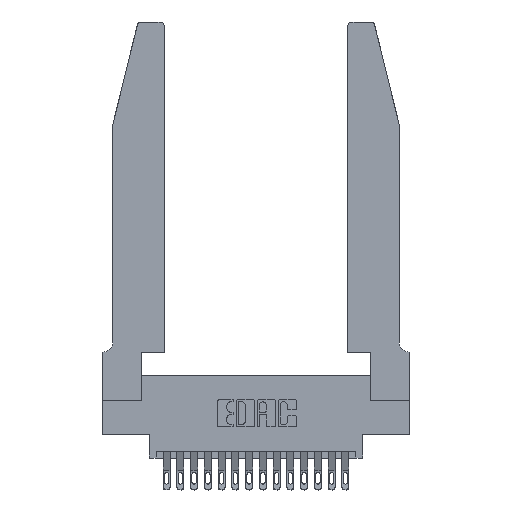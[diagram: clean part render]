
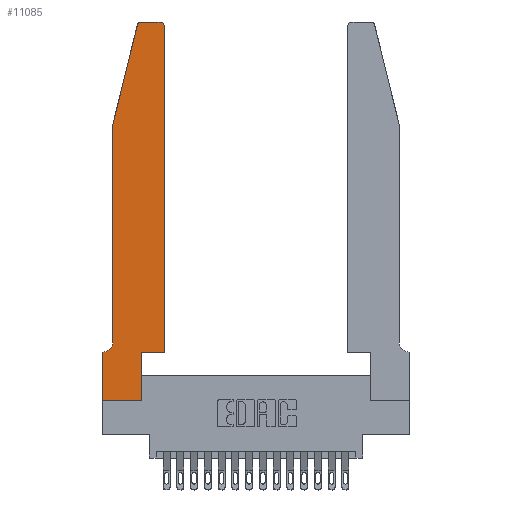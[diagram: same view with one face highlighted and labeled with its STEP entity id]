
A CAD part, top view. The second image highlights one B-rep face of the part: STEP entity #11085.
In plain terms, the highlighted planar face has unit normal (0, 0, 1).
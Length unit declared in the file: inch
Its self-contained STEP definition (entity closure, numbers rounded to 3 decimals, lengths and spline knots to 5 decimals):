
#4 = CARTESIAN_POINT ( 'NONE',  ( 0.4505, 2.72, 0.37 ) ) ;
#58 = CARTESIAN_POINT ( 'NONE',  ( 0.4505, 0.35, 0.37 ) ) ;
#345 = ORIENTED_EDGE ( 'NONE', *, *, #15492, .T. ) ;
#441 = DIRECTION ( 'NONE',  ( -1., 0., 0. ) ) ;
#541 = VERTEX_POINT ( 'NONE', #14167 ) ;
#592 = DIRECTION ( 'NONE',  ( 0., 1., 0. ) ) ;
#723 = CARTESIAN_POINT ( 'NONE',  ( 0.0055, 0.35, 0.37 ) ) ;
#910 = VERTEX_POINT ( 'NONE', #12138 ) ;
#1115 = AXIS2_PLACEMENT_3D ( 'NONE', #13196, #3932, #14712 ) ;
#1235 = DIRECTION ( 'NONE',  ( 1., 0., 0. ) ) ;
#1678 = CARTESIAN_POINT ( 'NONE',  ( 0., 0., 0.37 ) ) ;
#2380 = PLANE ( 'NONE',  #18724 ) ;
#2677 = LINE ( 'NONE', #18085, #17992 ) ;
#2682 = LINE ( 'NONE', #19079, #10477 ) ;
#2796 = EDGE_CURVE ( 'NONE', #14318, #12130, #13355, .T. ) ;
#2851 = DIRECTION ( 'NONE',  ( 0., 1., 0. ) ) ;
#2963 = EDGE_CURVE ( 'NONE', #10115, #4960, #7600, .T. ) ;
#3346 = DIRECTION ( 'NONE',  ( 1., 0., 0. ) ) ;
#3350 = EDGE_CURVE ( 'NONE', #5013, #13885, #16588, .T. ) ;
#3449 = CARTESIAN_POINT ( 'NONE',  ( 0.284, 2.75, 0.37 ) ) ;
#3913 = ORIENTED_EDGE ( 'NONE', *, *, #14777, .T. ) ;
#3932 = DIRECTION ( 'NONE',  ( 0., 0., -1. ) ) ;
#4013 = DIRECTION ( 'NONE',  ( 1., 0., 0. ) ) ;
#4354 = VECTOR ( 'NONE', #18451, 39.37008 ) ;
#4436 = VECTOR ( 'NONE', #9492, 39.37008 ) ;
#4551 = EDGE_CURVE ( 'NONE', #6329, #5013, #13321, .T. ) ;
#4612 = ORIENTED_EDGE ( 'NONE', *, *, #2963, .T. ) ;
#4767 = CARTESIAN_POINT ( 'NONE',  ( 0., 0.35, 0.37 ) ) ;
#4909 = ORIENTED_EDGE ( 'NONE', *, *, #10241, .T. ) ;
#4960 = VERTEX_POINT ( 'NONE', #723 ) ;
#5013 = VERTEX_POINT ( 'NONE', #8833 ) ;
#5078 = ORIENTED_EDGE ( 'NONE', *, *, #3350, .T. ) ;
#5857 = ORIENTED_EDGE ( 'NONE', *, *, #10189, .T. ) ;
#5964 = CARTESIAN_POINT ( 'NONE',  ( 0.284, 2.72, 0.37 ) ) ;
#6329 = VERTEX_POINT ( 'NONE', #3449 ) ;
#6366 = CARTESIAN_POINT ( 'NONE',  ( 0.0755, 0.35, 0.37 ) ) ;
#6390 = CARTESIAN_POINT ( 'NONE',  ( 0.4505, 0.35, 0.37 ) ) ;
#6743 = ORIENTED_EDGE ( 'NONE', *, *, #4551, .T. ) ;
#7114 = ORIENTED_EDGE ( 'NONE', *, *, #2796, .T. ) ;
#7282 = LINE ( 'NONE', #6390, #19296 ) ;
#7497 = DIRECTION ( 'NONE',  ( 1., 0., 0. ) ) ;
#7600 = CIRCLE ( 'NONE', #1115, 0.07 ) ;
#7942 = CARTESIAN_POINT ( 'NONE',  ( 0.0755, 2., 0.37 ) ) ;
#8217 = FACE_OUTER_BOUND ( 'NONE', #10931, .T. ) ;
#8408 = CARTESIAN_POINT ( 'NONE',  ( 0.0755, 2., 0.37 ) ) ;
#8461 = VERTEX_POINT ( 'NONE', #10868 ) ;
#8574 = VERTEX_POINT ( 'NONE', #58 ) ;
#8578 = CARTESIAN_POINT ( 'NONE',  ( 0.0755, 2., 0.37 ) ) ;
#8833 = CARTESIAN_POINT ( 'NONE',  ( 0.25487, 2.72718, 0.37 ) ) ;
#9206 = LINE ( 'NONE', #8578, #12765 ) ;
#9492 = DIRECTION ( 'NONE',  ( -0.239, -0.971, 0. ) ) ;
#9645 = VERTEX_POINT ( 'NONE', #4 ) ;
#9735 = VECTOR ( 'NONE', #15052, 39.37008 ) ;
#10003 = ORIENTED_EDGE ( 'NONE', *, *, #16224, .T. ) ;
#10101 = DIRECTION ( 'NONE',  ( 0., -1., 0. ) ) ;
#10115 = VERTEX_POINT ( 'NONE', #18274 ) ;
#10133 = AXIS2_PLACEMENT_3D ( 'NONE', #5964, #16564, #7497 ) ;
#10189 = EDGE_CURVE ( 'NONE', #541, #8574, #7282, .T. ) ;
#10241 = EDGE_CURVE ( 'NONE', #12130, #910, #10872, .T. ) ;
#10402 = VECTOR ( 'NONE', #3346, 39.37008 ) ;
#10477 = VECTOR ( 'NONE', #592, 39.37008 ) ;
#10629 = AXIS2_PLACEMENT_3D ( 'NONE', #19620, #10671, #1235 ) ;
#10671 = DIRECTION ( 'NONE',  ( 0., 0., 1. ) ) ;
#10836 = EDGE_CURVE ( 'NONE', #4960, #14318, #16522, .T. ) ;
#10868 = CARTESIAN_POINT ( 'NONE',  ( 0.4205, 2.75, 0.37 ) ) ;
#10872 = LINE ( 'NONE', #1678, #10402 ) ;
#10931 = EDGE_LOOP ( 'NONE', ( #14850, #6743, #5078, #12268, #4612, #11864, #7114, #4909, #345, #5857, #3913, #10003 ) ) ;
#11001 = VECTOR ( 'NONE', #441, 39.37008 ) ;
#11041 = EDGE_CURVE ( 'NONE', #13885, #10115, #9206, .T. ) ;
#11085 = ADVANCED_FACE ( 'NONE', ( #8217 ), #2380, .T. ) ;
#11481 = LINE ( 'NONE', #14512, #11001 ) ;
#11688 = CARTESIAN_POINT ( 'NONE',  ( 0., 0.35, 0.37 ) ) ;
#11864 = ORIENTED_EDGE ( 'NONE', *, *, #10836, .T. ) ;
#12130 = VERTEX_POINT ( 'NONE', #19112 ) ;
#12138 = CARTESIAN_POINT ( 'NONE',  ( 0.2865, 0., 0.37 ) ) ;
#12268 = ORIENTED_EDGE ( 'NONE', *, *, #11041, .T. ) ;
#12765 = VECTOR ( 'NONE', #10101, 39.37008 ) ;
#13196 = CARTESIAN_POINT ( 'NONE',  ( 0.0055, 0.42, 0.37 ) ) ;
#13280 = DIRECTION ( 'NONE',  ( 0., 0., 1. ) ) ;
#13321 = CIRCLE ( 'NONE', #10133, 0.03 ) ;
#13328 = EDGE_CURVE ( 'NONE', #8461, #6329, #11481, .T. ) ;
#13355 = LINE ( 'NONE', #16102, #9735 ) ;
#13885 = VERTEX_POINT ( 'NONE', #8408 ) ;
#14167 = CARTESIAN_POINT ( 'NONE',  ( 0.2865, 0.35, 0.37 ) ) ;
#14318 = VERTEX_POINT ( 'NONE', #4767 ) ;
#14512 = CARTESIAN_POINT ( 'NONE',  ( 0.2605, 2.75, 0.37 ) ) ;
#14712 = DIRECTION ( 'NONE',  ( -1., 0., 0. ) ) ;
#14777 = EDGE_CURVE ( 'NONE', #8574, #9645, #2677, .T. ) ;
#14850 = ORIENTED_EDGE ( 'NONE', *, *, #13328, .T. ) ;
#15052 = DIRECTION ( 'NONE',  ( 0., -1., 0. ) ) ;
#15492 = EDGE_CURVE ( 'NONE', #910, #541, #2682, .T. ) ;
#15549 = DIRECTION ( 'NONE',  ( 1., 0., 0. ) ) ;
#16102 = CARTESIAN_POINT ( 'NONE',  ( 0., 0., 0.37 ) ) ;
#16224 = EDGE_CURVE ( 'NONE', #9645, #8461, #17731, .T. ) ;
#16522 = LINE ( 'NONE', #6366, #4354 ) ;
#16564 = DIRECTION ( 'NONE',  ( 0., 0., 1. ) ) ;
#16588 = LINE ( 'NONE', #7942, #4436 ) ;
#17731 = CIRCLE ( 'NONE', #10629, 0.03 ) ;
#17992 = VECTOR ( 'NONE', #2851, 39.37008 ) ;
#18085 = CARTESIAN_POINT ( 'NONE',  ( 0.4505, 0.35, 0.37 ) ) ;
#18274 = CARTESIAN_POINT ( 'NONE',  ( 0.0755, 0.42, 0.37 ) ) ;
#18451 = DIRECTION ( 'NONE',  ( -1., 0., 0. ) ) ;
#18724 = AXIS2_PLACEMENT_3D ( 'NONE', #11688, #13280, #4013 ) ;
#19079 = CARTESIAN_POINT ( 'NONE',  ( 0.2865, 0.35, 0.37 ) ) ;
#19112 = CARTESIAN_POINT ( 'NONE',  ( 0., 0., 0.37 ) ) ;
#19296 = VECTOR ( 'NONE', #15549, 39.37008 ) ;
#19620 = CARTESIAN_POINT ( 'NONE',  ( 0.4205, 2.72, 0.37 ) ) ;
